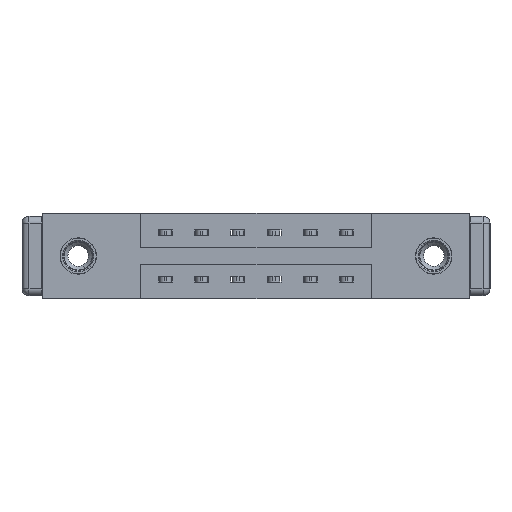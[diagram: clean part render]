
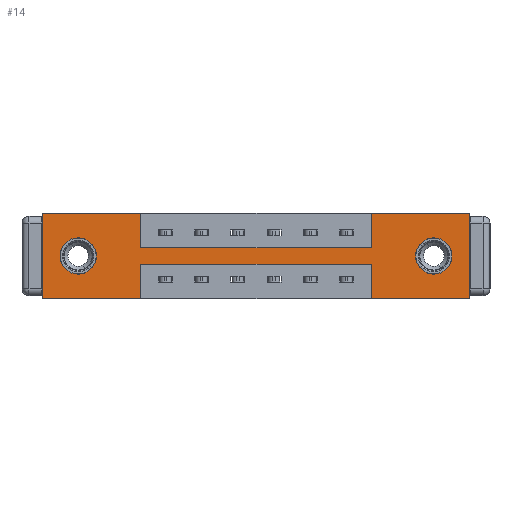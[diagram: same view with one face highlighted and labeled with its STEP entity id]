
A CAD part, front view. The second image highlights one B-rep face of the part: STEP entity #14.
In plain terms, the highlighted planar face has unit normal (0, -1, 0).
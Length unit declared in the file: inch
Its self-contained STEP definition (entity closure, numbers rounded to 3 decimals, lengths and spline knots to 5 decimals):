
#14 = ADVANCED_FACE ( 'NONE', ( #3344, #3492, #1431 ), #11844, .T. ) ;
#31 = EDGE_CURVE ( 'NONE', #277, #7831, #5502, .T. ) ;
#121 = CARTESIAN_POINT ( 'NONE',  ( 0.155, 0., -0.107 ) ) ;
#142 = CARTESIAN_POINT ( 'NONE',  ( 0., 0., -0.37 ) ) ;
#150 = VECTOR ( 'NONE', #8773, 39.37008 ) ;
#277 = VERTEX_POINT ( 'NONE', #2900 ) ;
#347 = EDGE_LOOP ( 'NONE', ( #5247, #4834 ) ) ;
#463 = CARTESIAN_POINT ( 'NONE',  ( 1.417, 0., -0.37 ) ) ;
#474 = CARTESIAN_POINT ( 'NONE',  ( 0.425, 0., 0. ) ) ;
#518 = AXIS2_PLACEMENT_3D ( 'NONE', #7281, #8152, #2585 ) ;
#600 = DIRECTION ( 'NONE',  ( 0., 0., -1. ) ) ;
#617 = CARTESIAN_POINT ( 'NONE',  ( 0.425, 0., -0.22 ) ) ;
#734 = CARTESIAN_POINT ( 'NONE',  ( 0.425, 0., -0.15 ) ) ;
#797 = DIRECTION ( 'NONE',  ( 1., 0., 0. ) ) ;
#835 = ORIENTED_EDGE ( 'NONE', *, *, #8147, .F. ) ;
#977 = DIRECTION ( 'NONE',  ( 1., 0., 0. ) ) ;
#982 = VERTEX_POINT ( 'NONE', #1805 ) ;
#1009 = ORIENTED_EDGE ( 'NONE', *, *, #4570, .T. ) ;
#1108 = DIRECTION ( 'NONE',  ( 0., 0., 1. ) ) ;
#1201 = ORIENTED_EDGE ( 'NONE', *, *, #6136, .F. ) ;
#1243 = CARTESIAN_POINT ( 'NONE',  ( 1.842, 0., -0.37 ) ) ;
#1255 = EDGE_CURVE ( 'NONE', #9079, #11204, #3607, .T. ) ;
#1390 = LINE ( 'NONE', #1562, #3175 ) ;
#1431 = FACE_OUTER_BOUND ( 'NONE', #6817, .T. ) ;
#1562 = CARTESIAN_POINT ( 'NONE',  ( 0.425, 0., -0.37 ) ) ;
#1574 = CARTESIAN_POINT ( 'NONE',  ( 1.687, 0., -0.263 ) ) ;
#1598 = EDGE_CURVE ( 'NONE', #2216, #2348, #8089, .T. ) ;
#1771 = CARTESIAN_POINT ( 'NONE',  ( 0.425, 0., -0.22 ) ) ;
#1792 = LINE ( 'NONE', #6700, #11408 ) ;
#1805 = CARTESIAN_POINT ( 'NONE',  ( 1.842, 0., 0. ) ) ;
#1818 = VECTOR ( 'NONE', #7142, 39.37008 ) ;
#1912 = EDGE_CURVE ( 'NONE', #2484, #7080, #1390, .T. ) ;
#1959 = ORIENTED_EDGE ( 'NONE', *, *, #7081, .F. ) ;
#1985 = CARTESIAN_POINT ( 'NONE',  ( 1.842, 0., 0. ) ) ;
#2216 = VERTEX_POINT ( 'NONE', #4231 ) ;
#2348 = VERTEX_POINT ( 'NONE', #1574 ) ;
#2469 = VECTOR ( 'NONE', #7685, 39.37008 ) ;
#2483 = CARTESIAN_POINT ( 'NONE',  ( 0., 0., -0.37 ) ) ;
#2484 = VERTEX_POINT ( 'NONE', #1771 ) ;
#2582 = CARTESIAN_POINT ( 'NONE',  ( 1.417, 0., -0.22 ) ) ;
#2585 = DIRECTION ( 'NONE',  ( 0., 0., 1. ) ) ;
#2650 = ORIENTED_EDGE ( 'NONE', *, *, #10314, .F. ) ;
#2823 = DIRECTION ( 'NONE',  ( -1., 0., 0. ) ) ;
#2900 = CARTESIAN_POINT ( 'NONE',  ( 0., 0., 0. ) ) ;
#3030 = DIRECTION ( 'NONE',  ( 0., 0., -1. ) ) ;
#3045 = ORIENTED_EDGE ( 'NONE', *, *, #6190, .F. ) ;
#3140 = LINE ( 'NONE', #7589, #8208 ) ;
#3148 = EDGE_CURVE ( 'NONE', #7080, #10548, #1792, .T. ) ;
#3175 = VECTOR ( 'NONE', #600, 39.37008 ) ;
#3268 = CARTESIAN_POINT ( 'NONE',  ( 0.155, 0., -0.263 ) ) ;
#3344 = FACE_BOUND ( 'NONE', #11031, .T. ) ;
#3357 = ORIENTED_EDGE ( 'NONE', *, *, #1912, .F. ) ;
#3492 = FACE_BOUND ( 'NONE', #347, .T. ) ;
#3607 = CIRCLE ( 'NONE', #518, 0.078 ) ;
#3680 = CARTESIAN_POINT ( 'NONE',  ( 0., 0., 0. ) ) ;
#3795 = CARTESIAN_POINT ( 'NONE',  ( 1.687, 0., -0.185 ) ) ;
#3911 = CARTESIAN_POINT ( 'NONE',  ( 1.417, 0., 0. ) ) ;
#3968 = CIRCLE ( 'NONE', #4259, 0.078 ) ;
#4091 = EDGE_CURVE ( 'NONE', #11204, #9079, #5832, .T. ) ;
#4098 = LINE ( 'NONE', #3680, #11223 ) ;
#4231 = CARTESIAN_POINT ( 'NONE',  ( 1.687, 0., -0.107 ) ) ;
#4259 = AXIS2_PLACEMENT_3D ( 'NONE', #3795, #4881, #4742 ) ;
#4265 = VERTEX_POINT ( 'NONE', #1243 ) ;
#4422 = ORIENTED_EDGE ( 'NONE', *, *, #31, .F. ) ;
#4570 = EDGE_CURVE ( 'NONE', #2348, #2216, #3968, .T. ) ;
#4713 = EDGE_CURVE ( 'NONE', #8984, #982, #4098, .T. ) ;
#4742 = DIRECTION ( 'NONE',  ( 0., 0., -1. ) ) ;
#4834 = ORIENTED_EDGE ( 'NONE', *, *, #1255, .T. ) ;
#4881 = DIRECTION ( 'NONE',  ( 0., 1., 0. ) ) ;
#5247 = ORIENTED_EDGE ( 'NONE', *, *, #4091, .T. ) ;
#5386 = DIRECTION ( 'NONE',  ( 0., 0., -1. ) ) ;
#5502 = LINE ( 'NONE', #10885, #7975 ) ;
#5522 = LINE ( 'NONE', #6647, #2469 ) ;
#5666 = VERTEX_POINT ( 'NONE', #9671 ) ;
#5832 = CIRCLE ( 'NONE', #10742, 0.078 ) ;
#5891 = DIRECTION ( 'NONE',  ( 0., 1., 0. ) ) ;
#5997 = CARTESIAN_POINT ( 'NONE',  ( 1.417, 0., -0.15 ) ) ;
#6004 = AXIS2_PLACEMENT_3D ( 'NONE', #9814, #9895, #6942 ) ;
#6136 = EDGE_CURVE ( 'NONE', #4265, #5666, #9402, .T. ) ;
#6190 = EDGE_CURVE ( 'NONE', #10548, #277, #10869, .T. ) ;
#6505 = EDGE_CURVE ( 'NONE', #9963, #2484, #8082, .T. ) ;
#6520 = DIRECTION ( 'NONE',  ( 0., 0., -1. ) ) ;
#6647 = CARTESIAN_POINT ( 'NONE',  ( 1.417, 0., 0. ) ) ;
#6700 = CARTESIAN_POINT ( 'NONE',  ( 0., 0., -0.37 ) ) ;
#6765 = VECTOR ( 'NONE', #2823, 39.37008 ) ;
#6817 = EDGE_LOOP ( 'NONE', ( #3357, #9136, #2650, #1201, #10381, #10613, #10485, #1959, #835, #4422, #3045, #7452 ) ) ;
#6942 = DIRECTION ( 'NONE',  ( 0., 0., -1. ) ) ;
#7080 = VERTEX_POINT ( 'NONE', #11897 ) ;
#7081 = EDGE_CURVE ( 'NONE', #8442, #8567, #7190, .T. ) ;
#7142 = DIRECTION ( 'NONE',  ( -1., 0., 0. ) ) ;
#7190 = LINE ( 'NONE', #734, #11565 ) ;
#7281 = CARTESIAN_POINT ( 'NONE',  ( 0.155, 0., -0.185 ) ) ;
#7452 = ORIENTED_EDGE ( 'NONE', *, *, #3148, .F. ) ;
#7589 = CARTESIAN_POINT ( 'NONE',  ( 0.425, 0., 0. ) ) ;
#7685 = DIRECTION ( 'NONE',  ( 0., 0., 1. ) ) ;
#7831 = VERTEX_POINT ( 'NONE', #474 ) ;
#7869 = VECTOR ( 'NONE', #6520, 39.37008 ) ;
#7975 = VECTOR ( 'NONE', #797, 39.37008 ) ;
#8082 = LINE ( 'NONE', #617, #1818 ) ;
#8089 = CIRCLE ( 'NONE', #6004, 0.078 ) ;
#8094 = VECTOR ( 'NONE', #1108, 39.37008 ) ;
#8147 = EDGE_CURVE ( 'NONE', #7831, #8442, #3140, .T. ) ;
#8152 = DIRECTION ( 'NONE',  ( 0., 1., 0. ) ) ;
#8207 = DIRECTION ( 'NONE',  ( 1., 0., 0. ) ) ;
#8208 = VECTOR ( 'NONE', #3030, 39.37008 ) ;
#8277 = DIRECTION ( 'NONE',  ( 0., -1., 0. ) ) ;
#8442 = VERTEX_POINT ( 'NONE', #10816 ) ;
#8567 = VERTEX_POINT ( 'NONE', #5997 ) ;
#8589 = AXIS2_PLACEMENT_3D ( 'NONE', #10959, #8277, #5386 ) ;
#8773 = DIRECTION ( 'NONE',  ( 0., 0., 1. ) ) ;
#8984 = VERTEX_POINT ( 'NONE', #3911 ) ;
#9079 = VERTEX_POINT ( 'NONE', #3268 ) ;
#9136 = ORIENTED_EDGE ( 'NONE', *, *, #6505, .F. ) ;
#9170 = LINE ( 'NONE', #1985, #7869 ) ;
#9402 = LINE ( 'NONE', #142, #6765 ) ;
#9574 = DIRECTION ( 'NONE',  ( -1., 0., 0. ) ) ;
#9619 = DIRECTION ( 'NONE',  ( 0., 0., 1. ) ) ;
#9661 = CARTESIAN_POINT ( 'NONE',  ( 0.155, 0., -0.185 ) ) ;
#9671 = CARTESIAN_POINT ( 'NONE',  ( 1.417, 0., -0.37 ) ) ;
#9814 = CARTESIAN_POINT ( 'NONE',  ( 1.687, 0., -0.185 ) ) ;
#9895 = DIRECTION ( 'NONE',  ( 0., 1., 0. ) ) ;
#9963 = VERTEX_POINT ( 'NONE', #2582 ) ;
#10061 = EDGE_CURVE ( 'NONE', #982, #4265, #9170, .T. ) ;
#10081 = ORIENTED_EDGE ( 'NONE', *, *, #1598, .T. ) ;
#10314 = EDGE_CURVE ( 'NONE', #5666, #9963, #10923, .T. ) ;
#10381 = ORIENTED_EDGE ( 'NONE', *, *, #10061, .F. ) ;
#10485 = ORIENTED_EDGE ( 'NONE', *, *, #10685, .F. ) ;
#10548 = VERTEX_POINT ( 'NONE', #2483 ) ;
#10603 = CARTESIAN_POINT ( 'NONE',  ( 0., 0., 0. ) ) ;
#10613 = ORIENTED_EDGE ( 'NONE', *, *, #4713, .F. ) ;
#10685 = EDGE_CURVE ( 'NONE', #8567, #8984, #5522, .T. ) ;
#10742 = AXIS2_PLACEMENT_3D ( 'NONE', #9661, #5891, #9619 ) ;
#10816 = CARTESIAN_POINT ( 'NONE',  ( 0.425, 0., -0.15 ) ) ;
#10869 = LINE ( 'NONE', #10603, #8094 ) ;
#10885 = CARTESIAN_POINT ( 'NONE',  ( 0., 0., 0. ) ) ;
#10923 = LINE ( 'NONE', #463, #150 ) ;
#10959 = CARTESIAN_POINT ( 'NONE',  ( 0., 0., -0.37 ) ) ;
#11031 = EDGE_LOOP ( 'NONE', ( #10081, #1009 ) ) ;
#11204 = VERTEX_POINT ( 'NONE', #121 ) ;
#11223 = VECTOR ( 'NONE', #977, 39.37008 ) ;
#11408 = VECTOR ( 'NONE', #9574, 39.37008 ) ;
#11565 = VECTOR ( 'NONE', #8207, 39.37008 ) ;
#11844 = PLANE ( 'NONE',  #8589 ) ;
#11897 = CARTESIAN_POINT ( 'NONE',  ( 0.425, 0., -0.37 ) ) ;
